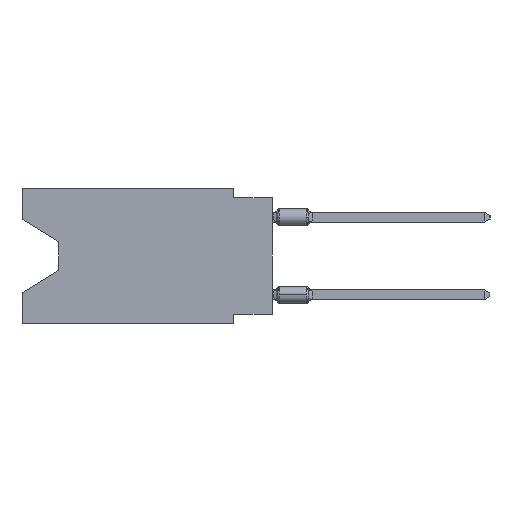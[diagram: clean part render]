
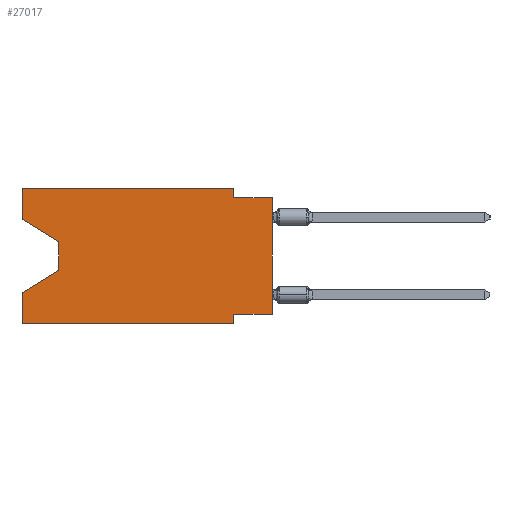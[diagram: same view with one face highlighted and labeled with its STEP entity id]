
A CAD part, left-side view. The second image highlights one B-rep face of the part: STEP entity #27017.
In plain terms, the highlighted planar face has unit normal (-1, 0, 0).
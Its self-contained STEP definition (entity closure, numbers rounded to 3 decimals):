
#138 = DIRECTION ( 'NONE',  ( 0., 0., 1. ) ) ;
#386 = EDGE_CURVE ( 'NONE', #854, #39944, #13076, .T. ) ;
#854 = VERTEX_POINT ( 'NONE', #33803 ) ;
#1013 = DIRECTION ( 'NONE',  ( 0., 0., -1. ) ) ;
#3158 = ORIENTED_EDGE ( 'NONE', *, *, #33925, .F. ) ;
#5409 = CARTESIAN_POINT ( 'NONE',  ( 0., 2.54, -0.635 ) ) ;
#5671 = DIRECTION ( 'NONE',  ( 0., 0., -1. ) ) ;
#6195 = CARTESIAN_POINT ( 'NONE',  ( 0., 13.97, -5.385 ) ) ;
#7811 = VECTOR ( 'NONE', #5671, 1000. ) ;
#7883 = LINE ( 'NONE', #35807, #16434 ) ;
#8597 = ORIENTED_EDGE ( 'NONE', *, *, #35219, .F. ) ;
#8681 = EDGE_CURVE ( 'NONE', #25787, #42435, #34555, .T. ) ;
#8693 = VECTOR ( 'NONE', #27030, 1000. ) ;
#9789 = VECTOR ( 'NONE', #45001, 1000. ) ;
#9824 = EDGE_CURVE ( 'NONE', #854, #42435, #21036, .T. ) ;
#9843 = ORIENTED_EDGE ( 'NONE', *, *, #12533, .T. ) ;
#9850 = DIRECTION ( 'NONE',  ( 0., -0.855, -0.519 ) ) ;
#10077 = VECTOR ( 'NONE', #35914, 1000. ) ;
#10334 = CARTESIAN_POINT ( 'NONE',  ( 0., 13.97, -3.505 ) ) ;
#10526 = VERTEX_POINT ( 'NONE', #10334 ) ;
#11169 = CARTESIAN_POINT ( 'NONE',  ( 0., 16.383, 0. ) ) ;
#11765 = LINE ( 'NONE', #21842, #33156 ) ;
#11910 = EDGE_LOOP ( 'NONE', ( #44075, #9843, #26162, #17740, #12132, #42079, #18260, #30092, #3158, #19988, #8597, #25722 ) ) ;
#12132 = ORIENTED_EDGE ( 'NONE', *, *, #386, .T. ) ;
#12533 = EDGE_CURVE ( 'NONE', #10526, #25787, #40427, .T. ) ;
#12968 = VECTOR ( 'NONE', #31885, 1000. ) ;
#13001 = VERTEX_POINT ( 'NONE', #44262 ) ;
#13076 = LINE ( 'NONE', #40283, #8693 ) ;
#13602 = DIRECTION ( 'NONE',  ( 1., 0., 0. ) ) ;
#13800 = LINE ( 'NONE', #18114, #33182 ) ;
#14835 = CARTESIAN_POINT ( 'NONE',  ( 0., 16.383, -6.852 ) ) ;
#15053 = CARTESIAN_POINT ( 'NONE',  ( 0., 2.54, -8.255 ) ) ;
#15328 = DIRECTION ( 'NONE',  ( 0., 1., 0. ) ) ;
#15560 = VERTEX_POINT ( 'NONE', #42612 ) ;
#16434 = VECTOR ( 'NONE', #1013, 1000. ) ;
#16987 = VERTEX_POINT ( 'NONE', #36107 ) ;
#17174 = CARTESIAN_POINT ( 'NONE',  ( 0., 13.97, -5.385 ) ) ;
#17475 = PLANE ( 'NONE',  #32281 ) ;
#17740 = ORIENTED_EDGE ( 'NONE', *, *, #9824, .F. ) ;
#17922 = CARTESIAN_POINT ( 'NONE',  ( 0., 0., -0.635 ) ) ;
#18052 = VERTEX_POINT ( 'NONE', #35033 ) ;
#18114 = CARTESIAN_POINT ( 'NONE',  ( 0., 16.383, 0. ) ) ;
#18260 = ORIENTED_EDGE ( 'NONE', *, *, #38367, .F. ) ;
#18609 = VECTOR ( 'NONE', #9850, 1000. ) ;
#19988 = ORIENTED_EDGE ( 'NONE', *, *, #34504, .F. ) ;
#20525 = CARTESIAN_POINT ( 'NONE',  ( 0., 13.97, -3.505 ) ) ;
#20670 = CARTESIAN_POINT ( 'NONE',  ( 0., 16.383, 0. ) ) ;
#21036 = LINE ( 'NONE', #11169, #28446 ) ;
#21262 = DIRECTION ( 'NONE',  ( 0., 0., 1. ) ) ;
#21349 = DIRECTION ( 'NONE',  ( 0., 0., -1. ) ) ;
#21842 = CARTESIAN_POINT ( 'NONE',  ( 0., 0., 0. ) ) ;
#24229 = VECTOR ( 'NONE', #15328, 1000. ) ;
#24562 = FACE_OUTER_BOUND ( 'NONE', #11910, .T. ) ;
#25346 = VECTOR ( 'NONE', #138, 1000. ) ;
#25360 = EDGE_CURVE ( 'NONE', #39562, #39944, #7883, .T. ) ;
#25722 = ORIENTED_EDGE ( 'NONE', *, *, #33463, .F. ) ;
#25787 = VERTEX_POINT ( 'NONE', #6195 ) ;
#26075 = LINE ( 'NONE', #35917, #24229 ) ;
#26162 = ORIENTED_EDGE ( 'NONE', *, *, #8681, .T. ) ;
#27017 = ADVANCED_FACE ( 'NONE', ( #24562 ), #17475, .F. ) ;
#27030 = DIRECTION ( 'NONE',  ( 0., -1., 0. ) ) ;
#27165 = LINE ( 'NONE', #32957, #9789 ) ;
#27570 = LINE ( 'NONE', #17922, #12968 ) ;
#28446 = VECTOR ( 'NONE', #21262, 1000. ) ;
#30092 = ORIENTED_EDGE ( 'NONE', *, *, #30536, .T. ) ;
#30536 = EDGE_CURVE ( 'NONE', #15560, #18052, #11765, .T. ) ;
#31885 = DIRECTION ( 'NONE',  ( 0., -1., 0. ) ) ;
#32281 = AXIS2_PLACEMENT_3D ( 'NONE', #20670, #13602, #21349 ) ;
#32957 = CARTESIAN_POINT ( 'NONE',  ( 0., 2.54, 0. ) ) ;
#33156 = VECTOR ( 'NONE', #39215, 1000. ) ;
#33182 = VECTOR ( 'NONE', #35268, 1000. ) ;
#33463 = EDGE_CURVE ( 'NONE', #41375, #13001, #34925, .T. ) ;
#33803 = CARTESIAN_POINT ( 'NONE',  ( 0., 16.383, -8.89 ) ) ;
#33925 = EDGE_CURVE ( 'NONE', #45114, #18052, #27570, .T. ) ;
#34504 = EDGE_CURVE ( 'NONE', #16987, #45114, #27165, .T. ) ;
#34555 = LINE ( 'NONE', #17174, #10077 ) ;
#34925 = LINE ( 'NONE', #38353, #25346 ) ;
#35033 = CARTESIAN_POINT ( 'NONE',  ( 0., 0., -0.635 ) ) ;
#35219 = EDGE_CURVE ( 'NONE', #13001, #16987, #13800, .T. ) ;
#35268 = DIRECTION ( 'NONE',  ( 0., -1., 0. ) ) ;
#35807 = CARTESIAN_POINT ( 'NONE',  ( 0., 2.54, -8.89 ) ) ;
#35914 = DIRECTION ( 'NONE',  ( 0., 0.855, -0.519 ) ) ;
#35917 = CARTESIAN_POINT ( 'NONE',  ( 0., 0., -8.255 ) ) ;
#36107 = CARTESIAN_POINT ( 'NONE',  ( 0., 2.54, 0. ) ) ;
#36714 = EDGE_CURVE ( 'NONE', #41375, #10526, #44624, .T. ) ;
#36788 = CARTESIAN_POINT ( 'NONE',  ( 0., 16.383, -2.038 ) ) ;
#37094 = CARTESIAN_POINT ( 'NONE',  ( 0., 16.383, -2.038 ) ) ;
#38353 = CARTESIAN_POINT ( 'NONE',  ( 0., 16.383, 0. ) ) ;
#38367 = EDGE_CURVE ( 'NONE', #15560, #39562, #26075, .T. ) ;
#39215 = DIRECTION ( 'NONE',  ( 0., 0., 1. ) ) ;
#39243 = CARTESIAN_POINT ( 'NONE',  ( 0., 2.54, -8.89 ) ) ;
#39562 = VERTEX_POINT ( 'NONE', #15053 ) ;
#39944 = VERTEX_POINT ( 'NONE', #39243 ) ;
#40283 = CARTESIAN_POINT ( 'NONE',  ( 0., 16.383, -8.89 ) ) ;
#40427 = LINE ( 'NONE', #20525, #7811 ) ;
#41375 = VERTEX_POINT ( 'NONE', #36788 ) ;
#42079 = ORIENTED_EDGE ( 'NONE', *, *, #25360, .F. ) ;
#42435 = VERTEX_POINT ( 'NONE', #14835 ) ;
#42612 = CARTESIAN_POINT ( 'NONE',  ( 0., 0., -8.255 ) ) ;
#44075 = ORIENTED_EDGE ( 'NONE', *, *, #36714, .T. ) ;
#44262 = CARTESIAN_POINT ( 'NONE',  ( 0., 16.383, 0. ) ) ;
#44624 = LINE ( 'NONE', #37094, #18609 ) ;
#45001 = DIRECTION ( 'NONE',  ( 0., 0., -1. ) ) ;
#45114 = VERTEX_POINT ( 'NONE', #5409 ) ;
